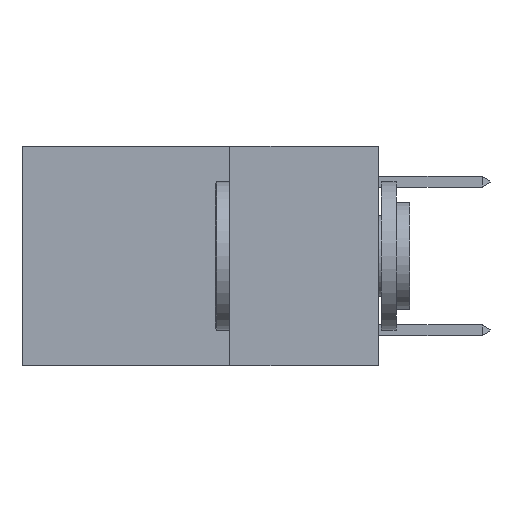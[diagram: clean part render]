
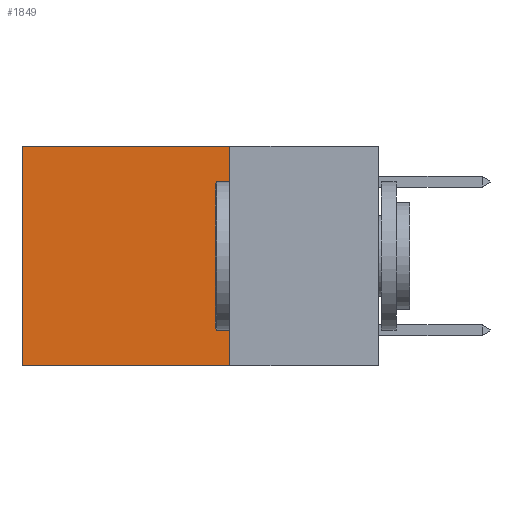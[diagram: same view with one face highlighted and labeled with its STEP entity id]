
A CAD part, left-side view. The second image highlights one B-rep face of the part: STEP entity #1849.
In plain terms, the highlighted planar face has unit normal (-1, 0, 0).
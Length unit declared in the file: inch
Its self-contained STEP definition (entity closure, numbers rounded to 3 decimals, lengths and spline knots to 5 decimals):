
#754 = VECTOR ( 'NONE', #17293, 39.37008 ) ;
#1459 = EDGE_CURVE ( 'NONE', #6664, #14520, #17796, .T. ) ;
#1849 = ADVANCED_FACE ( 'NONE', ( #7229 ), #2708, .F. ) ;
#2708 = PLANE ( 'NONE',  #13889 ) ;
#2750 = EDGE_CURVE ( 'NONE', #23020, #6664, #19331, .T. ) ;
#2952 = EDGE_CURVE ( 'NONE', #23020, #7069, #29235, .T. ) ;
#2960 = CARTESIAN_POINT ( 'NONE',  ( 0.2625, 0.6, -0.37 ) ) ;
#2995 = CARTESIAN_POINT ( 'NONE',  ( 0.2625, 0.25, 0. ) ) ;
#3763 = EDGE_LOOP ( 'NONE', ( #8021, #19698, #16869, #9948 ) ) ;
#6371 = DIRECTION ( 'NONE',  ( 0., 0., -1. ) ) ;
#6664 = VERTEX_POINT ( 'NONE', #20841 ) ;
#7069 = VERTEX_POINT ( 'NONE', #21666 ) ;
#7112 = VECTOR ( 'NONE', #9854, 39.37008 ) ;
#7229 = FACE_OUTER_BOUND ( 'NONE', #3763, .T. ) ;
#8021 = ORIENTED_EDGE ( 'NONE', *, *, #1459, .T. ) ;
#8136 = CARTESIAN_POINT ( 'NONE',  ( 0.2625, 0.25, -0.37 ) ) ;
#8572 = VECTOR ( 'NONE', #6371, 39.37008 ) ;
#9786 = LINE ( 'NONE', #8136, #754 ) ;
#9854 = DIRECTION ( 'NONE',  ( 0., 1., 0. ) ) ;
#9948 = ORIENTED_EDGE ( 'NONE', *, *, #2750, .T. ) ;
#11190 = CARTESIAN_POINT ( 'NONE',  ( 0.2625, 0.25, 0. ) ) ;
#13889 = AXIS2_PLACEMENT_3D ( 'NONE', #2995, #19244, #16381 ) ;
#14520 = VERTEX_POINT ( 'NONE', #2960 ) ;
#14673 = CARTESIAN_POINT ( 'NONE',  ( 0.2625, 0.25, 0. ) ) ;
#16381 = DIRECTION ( 'NONE',  ( 0., 0., -1. ) ) ;
#16869 = ORIENTED_EDGE ( 'NONE', *, *, #2952, .F. ) ;
#17293 = DIRECTION ( 'NONE',  ( 0., 1., 0. ) ) ;
#17796 = LINE ( 'NONE', #18394, #8572 ) ;
#18394 = CARTESIAN_POINT ( 'NONE',  ( 0.2625, 0.6, 0. ) ) ;
#19244 = DIRECTION ( 'NONE',  ( 1., 0., 0. ) ) ;
#19331 = LINE ( 'NONE', #14673, #7112 ) ;
#19698 = ORIENTED_EDGE ( 'NONE', *, *, #20670, .F. ) ;
#19770 = DIRECTION ( 'NONE',  ( 0., 0., -1. ) ) ;
#20670 = EDGE_CURVE ( 'NONE', #7069, #14520, #9786, .T. ) ;
#20841 = CARTESIAN_POINT ( 'NONE',  ( 0.2625, 0.6, 0. ) ) ;
#21666 = CARTESIAN_POINT ( 'NONE',  ( 0.2625, 0.25, -0.37 ) ) ;
#23020 = VERTEX_POINT ( 'NONE', #27289 ) ;
#27289 = CARTESIAN_POINT ( 'NONE',  ( 0.2625, 0.25, 0. ) ) ;
#27309 = VECTOR ( 'NONE', #19770, 39.37008 ) ;
#29235 = LINE ( 'NONE', #11190, #27309 ) ;
